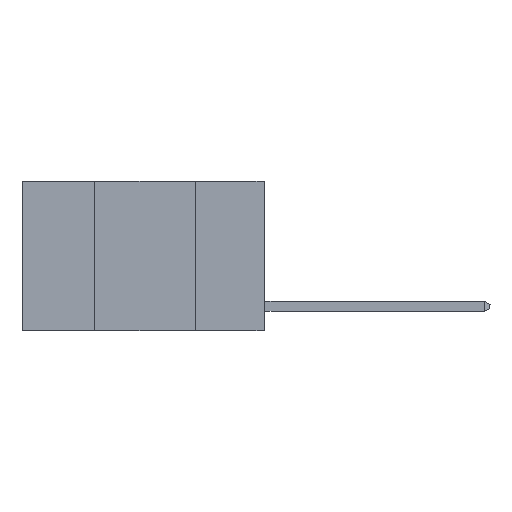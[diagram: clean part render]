
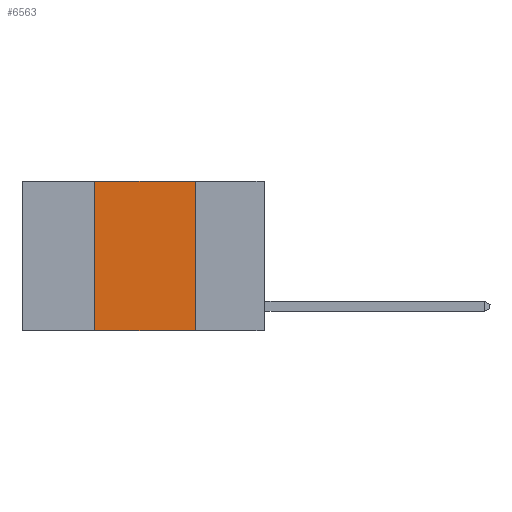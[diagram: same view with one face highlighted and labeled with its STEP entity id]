
A CAD part, left-side view. The second image highlights one B-rep face of the part: STEP entity #6563.
In plain terms, the highlighted planar face has unit normal (-1, 0, 0).
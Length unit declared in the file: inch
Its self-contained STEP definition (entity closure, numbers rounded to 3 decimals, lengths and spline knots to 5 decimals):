
#1361 = CARTESIAN_POINT ( 'NONE',  ( 0., 0.17, 0. ) ) ;
#1372 = CARTESIAN_POINT ( 'NONE',  ( 0., 0.6, -0.37 ) ) ;
#1416 = CARTESIAN_POINT ( 'NONE',  ( 0., 0.17, 0. ) ) ;
#1547 = CARTESIAN_POINT ( 'NONE',  ( 0., 0.17, -0.37 ) ) ;
#1737 = ORIENTED_EDGE ( 'NONE', *, *, #6179, .T. ) ;
#2171 = VECTOR ( 'NONE', #6529, 39.37008 ) ;
#2281 = VECTOR ( 'NONE', #8425, 39.37008 ) ;
#2557 = ORIENTED_EDGE ( 'NONE', *, *, #6923, .F. ) ;
#3106 = EDGE_CURVE ( 'NONE', #11023, #8000, #4543, .T. ) ;
#3193 = LINE ( 'NONE', #1416, #10837 ) ;
#3403 = EDGE_LOOP ( 'NONE', ( #3616, #7516, #2557, #1737 ) ) ;
#3616 = ORIENTED_EDGE ( 'NONE', *, *, #4699, .F. ) ;
#3780 = LINE ( 'NONE', #9386, #2281 ) ;
#3793 = FACE_OUTER_BOUND ( 'NONE', #3403, .T. ) ;
#3843 = PLANE ( 'NONE',  #8912 ) ;
#4543 = LINE ( 'NONE', #9209, #2171 ) ;
#4644 = CARTESIAN_POINT ( 'NONE',  ( 0., 0.42, 0. ) ) ;
#4699 = EDGE_CURVE ( 'NONE', #8000, #10834, #3193, .T. ) ;
#5137 = DIRECTION ( 'NONE',  ( 0., 0., -1. ) ) ;
#5264 = VECTOR ( 'NONE', #9642, 39.37008 ) ;
#5376 = VERTEX_POINT ( 'NONE', #6045 ) ;
#6045 = CARTESIAN_POINT ( 'NONE',  ( 0., 0.42, -0.37 ) ) ;
#6179 = EDGE_CURVE ( 'NONE', #5376, #10834, #7898, .T. ) ;
#6529 = DIRECTION ( 'NONE',  ( 0., -1., 0. ) ) ;
#6563 = ADVANCED_FACE ( 'NONE', ( #3793 ), #3843, .F. ) ;
#6923 = EDGE_CURVE ( 'NONE', #5376, #11023, #3780, .T. ) ;
#7516 = ORIENTED_EDGE ( 'NONE', *, *, #3106, .F. ) ;
#7581 = CARTESIAN_POINT ( 'NONE',  ( 0., 0.6, 0. ) ) ;
#7898 = LINE ( 'NONE', #1372, #5264 ) ;
#8000 = VERTEX_POINT ( 'NONE', #1361 ) ;
#8425 = DIRECTION ( 'NONE',  ( 0., 0., 1. ) ) ;
#8542 = DIRECTION ( 'NONE',  ( 1., 0., 0. ) ) ;
#8912 = AXIS2_PLACEMENT_3D ( 'NONE', #7581, #8542, #11291 ) ;
#9209 = CARTESIAN_POINT ( 'NONE',  ( 0., 0.6, 0. ) ) ;
#9386 = CARTESIAN_POINT ( 'NONE',  ( 0., 0.42, 0. ) ) ;
#9642 = DIRECTION ( 'NONE',  ( 0., -1., 0. ) ) ;
#10834 = VERTEX_POINT ( 'NONE', #1547 ) ;
#10837 = VECTOR ( 'NONE', #5137, 39.37008 ) ;
#11023 = VERTEX_POINT ( 'NONE', #4644 ) ;
#11291 = DIRECTION ( 'NONE',  ( 0., 0., -1. ) ) ;
